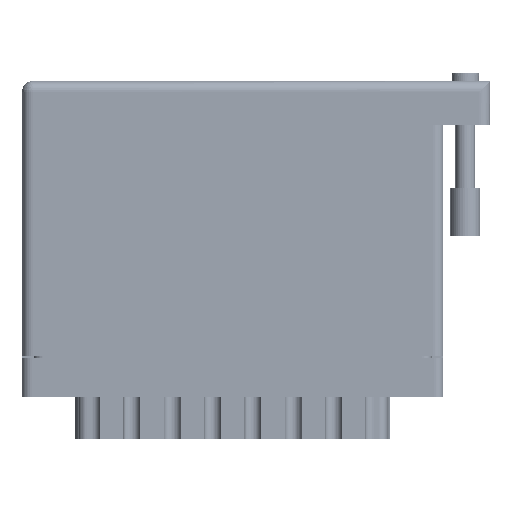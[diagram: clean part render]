
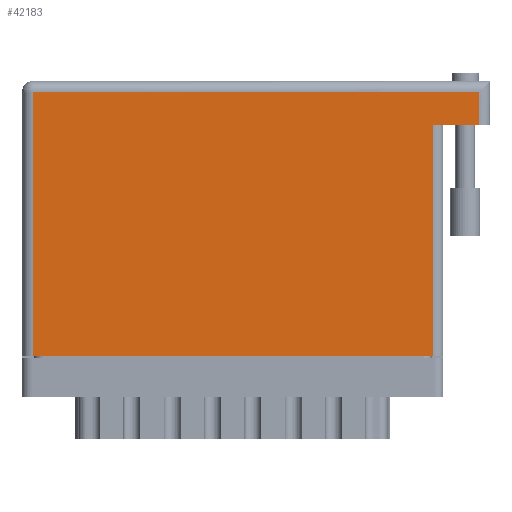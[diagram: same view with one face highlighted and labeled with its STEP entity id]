
A CAD part, front view. The second image highlights one B-rep face of the part: STEP entity #42183.
In plain terms, the highlighted face is planar.
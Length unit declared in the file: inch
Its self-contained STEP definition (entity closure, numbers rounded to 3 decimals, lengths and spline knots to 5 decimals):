
#649 = EDGE_CURVE ( 'NONE', #39909, #69255, #39348, .T. ) ;
#2172 = CARTESIAN_POINT ( 'NONE',  ( 2.648, 1.495, 0. ) ) ;
#3802 = DIRECTION ( 'NONE',  ( 0., 1., 0. ) ) ;
#4241 = VECTOR ( 'NONE', #9874, 39.37008 ) ;
#4551 = CARTESIAN_POINT ( 'NONE',  ( 2.948, 1.705, 0. ) ) ;
#7570 = VERTEX_POINT ( 'NONE', #43517 ) ;
#9223 = CARTESIAN_POINT ( 'NONE',  ( 0.07, 1.705, 0. ) ) ;
#9874 = DIRECTION ( 'NONE',  ( 0., -1., 0. ) ) ;
#10897 = PLANE ( 'NONE',  #17374 ) ;
#12505 = ORIENTED_EDGE ( 'NONE', *, *, #65266, .T. ) ;
#13038 = DIRECTION ( 'NONE',  ( 0., 1., 0. ) ) ;
#13359 = LINE ( 'NONE', #57005, #35303 ) ;
#14021 = EDGE_CURVE ( 'NONE', #69255, #7570, #62624, .T. ) ;
#14458 = LINE ( 'NONE', #43086, #19766 ) ;
#15554 = CARTESIAN_POINT ( 'NONE',  ( 0., 1.705, 0. ) ) ;
#16060 = DIRECTION ( 'NONE',  ( -1., 0., 0. ) ) ;
#17374 = AXIS2_PLACEMENT_3D ( 'NONE', #27827, #49164, #16060 ) ;
#17785 = VECTOR ( 'NONE', #71927, 39.37008 ) ;
#19766 = VECTOR ( 'NONE', #20805, 39.37008 ) ;
#20805 = DIRECTION ( 'NONE',  ( -1., 0., 0. ) ) ;
#21085 = CARTESIAN_POINT ( 'NONE',  ( 2.948, 1.775, 0. ) ) ;
#23738 = EDGE_CURVE ( 'NONE', #38158, #39909, #32678, .T. ) ;
#26416 = ORIENTED_EDGE ( 'NONE', *, *, #14021, .T. ) ;
#27110 = FACE_OUTER_BOUND ( 'NONE', #70195, .T. ) ;
#27827 = CARTESIAN_POINT ( 'NONE',  ( 0., 1.775, 0. ) ) ;
#30566 = CARTESIAN_POINT ( 'NONE',  ( 0.07, 0., 0. ) ) ;
#32678 = LINE ( 'NONE', #15554, #17785 ) ;
#35303 = VECTOR ( 'NONE', #13038, 39.37008 ) ;
#35591 = EDGE_CURVE ( 'NONE', #67440, #70444, #14458, .T. ) ;
#38158 = VERTEX_POINT ( 'NONE', #4551 ) ;
#39348 = LINE ( 'NONE', #65534, #4241 ) ;
#39909 = VERTEX_POINT ( 'NONE', #9223 ) ;
#42183 = ADVANCED_FACE ( 'NONE', ( #27110 ), #10897, .F. ) ;
#42345 = DIRECTION ( 'NONE',  ( 1., 0., 0. ) ) ;
#42732 = ORIENTED_EDGE ( 'NONE', *, *, #649, .T. ) ;
#43086 = CARTESIAN_POINT ( 'NONE',  ( 3.018, 1.495, 0. ) ) ;
#43517 = CARTESIAN_POINT ( 'NONE',  ( 2.648, 0., 0. ) ) ;
#47027 = VECTOR ( 'NONE', #3802, 39.37008 ) ;
#48716 = CARTESIAN_POINT ( 'NONE',  ( 0., 0., 0. ) ) ;
#49164 = DIRECTION ( 'NONE',  ( 0., 0., -1. ) ) ;
#54100 = LINE ( 'NONE', #21085, #47027 ) ;
#57005 = CARTESIAN_POINT ( 'NONE',  ( 2.648, 1.495, 0. ) ) ;
#58860 = ORIENTED_EDGE ( 'NONE', *, *, #23738, .T. ) ;
#60826 = ORIENTED_EDGE ( 'NONE', *, *, #35591, .F. ) ;
#62624 = LINE ( 'NONE', #48716, #63479 ) ;
#63479 = VECTOR ( 'NONE', #42345, 39.37008 ) ;
#64381 = ORIENTED_EDGE ( 'NONE', *, *, #72014, .T. ) ;
#65266 = EDGE_CURVE ( 'NONE', #7570, #70444, #13359, .T. ) ;
#65268 = CARTESIAN_POINT ( 'NONE',  ( 2.948, 1.495, 0. ) ) ;
#65534 = CARTESIAN_POINT ( 'NONE',  ( 0.07, 0., 0. ) ) ;
#67440 = VERTEX_POINT ( 'NONE', #65268 ) ;
#69255 = VERTEX_POINT ( 'NONE', #30566 ) ;
#70195 = EDGE_LOOP ( 'NONE', ( #26416, #12505, #60826, #64381, #58860, #42732 ) ) ;
#70444 = VERTEX_POINT ( 'NONE', #2172 ) ;
#71927 = DIRECTION ( 'NONE',  ( -1., 0., 0. ) ) ;
#72014 = EDGE_CURVE ( 'NONE', #67440, #38158, #54100, .T. ) ;
